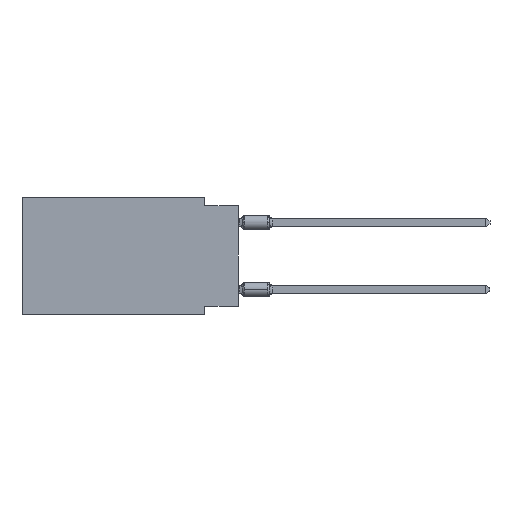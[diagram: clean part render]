
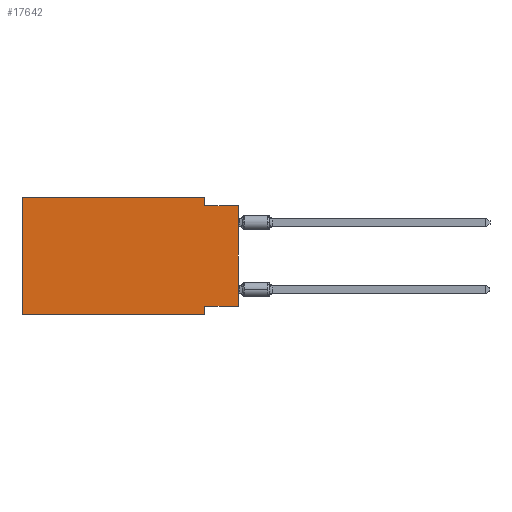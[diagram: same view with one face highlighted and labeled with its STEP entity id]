
A CAD part, left-side view. The second image highlights one B-rep face of the part: STEP entity #17642.
In plain terms, the highlighted planar face has unit normal (-1, 0, 0).
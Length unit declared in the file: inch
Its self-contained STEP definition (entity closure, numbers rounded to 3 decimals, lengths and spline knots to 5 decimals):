
#268 = VECTOR ( 'NONE', #18436, 39.37008 ) ;
#1188 = CARTESIAN_POINT ( 'NONE',  ( 0., 0.645, -0.35 ) ) ;
#1792 = VECTOR ( 'NONE', #5262, 39.37008 ) ;
#1881 = DIRECTION ( 'NONE',  ( 0., 0., -1. ) ) ;
#2581 = CARTESIAN_POINT ( 'NONE',  ( 0., 0.645, 0. ) ) ;
#3119 = DIRECTION ( 'NONE',  ( 0., -1., 0. ) ) ;
#3482 = ORIENTED_EDGE ( 'NONE', *, *, #6467, .T. ) ;
#3500 = CARTESIAN_POINT ( 'NONE',  ( 0., 0., 0. ) ) ;
#3630 = EDGE_CURVE ( 'NONE', #13139, #17908, #11127, .T. ) ;
#3745 = CARTESIAN_POINT ( 'NONE',  ( 0., 0.645, 0. ) ) ;
#5262 = DIRECTION ( 'NONE',  ( 0., 0., 1. ) ) ;
#5352 = ORIENTED_EDGE ( 'NONE', *, *, #11993, .F. ) ;
#6330 = CARTESIAN_POINT ( 'NONE',  ( 0., 0.1, 0. ) ) ;
#6467 = EDGE_CURVE ( 'NONE', #12580, #21857, #8977, .T. ) ;
#6472 = DIRECTION ( 'NONE',  ( 0., 0., 1. ) ) ;
#6615 = VECTOR ( 'NONE', #6472, 39.37008 ) ;
#6706 = VERTEX_POINT ( 'NONE', #23447 ) ;
#6881 = EDGE_CURVE ( 'NONE', #12580, #21814, #10828, .T. ) ;
#7970 = LINE ( 'NONE', #6330, #20561 ) ;
#8062 = EDGE_CURVE ( 'NONE', #13139, #24578, #14453, .T. ) ;
#8977 = LINE ( 'NONE', #16486, #16970 ) ;
#8992 = ORIENTED_EDGE ( 'NONE', *, *, #3630, .T. ) ;
#9120 = ORIENTED_EDGE ( 'NONE', *, *, #24662, .F. ) ;
#9430 = ORIENTED_EDGE ( 'NONE', *, *, #8062, .F. ) ;
#9650 = DIRECTION ( 'NONE',  ( 0., -1., 0. ) ) ;
#9866 = CARTESIAN_POINT ( 'NONE',  ( 0., 0., -0.025 ) ) ;
#10828 = LINE ( 'NONE', #20180, #6615 ) ;
#10831 = CARTESIAN_POINT ( 'NONE',  ( 0., 0., -0.325 ) ) ;
#10899 = EDGE_LOOP ( 'NONE', ( #8992, #5352, #17950, #16220, #21722, #3482, #9120, #9430 ) ) ;
#11127 = LINE ( 'NONE', #3500, #1792 ) ;
#11604 = EDGE_CURVE ( 'NONE', #21814, #18678, #19053, .T. ) ;
#11606 = DIRECTION ( 'NONE',  ( 1., 0., 0. ) ) ;
#11798 = DIRECTION ( 'NONE',  ( 0., 0., -1. ) ) ;
#11922 = CARTESIAN_POINT ( 'NONE',  ( 0., 0.1, 0. ) ) ;
#11942 = CARTESIAN_POINT ( 'NONE',  ( 0., 0.1, -0.35 ) ) ;
#11993 = EDGE_CURVE ( 'NONE', #6706, #17908, #13275, .T. ) ;
#12474 = EDGE_CURVE ( 'NONE', #18678, #6706, #7970, .T. ) ;
#12580 = VERTEX_POINT ( 'NONE', #1188 ) ;
#12879 = DIRECTION ( 'NONE',  ( 0., 0., -1. ) ) ;
#13128 = PLANE ( 'NONE',  #24532 ) ;
#13139 = VERTEX_POINT ( 'NONE', #17342 ) ;
#13275 = LINE ( 'NONE', #13401, #22960 ) ;
#13401 = CARTESIAN_POINT ( 'NONE',  ( 0., 0., -0.025 ) ) ;
#14453 = LINE ( 'NONE', #10831, #268 ) ;
#16220 = ORIENTED_EDGE ( 'NONE', *, *, #11604, .F. ) ;
#16486 = CARTESIAN_POINT ( 'NONE',  ( 0., 0.645, -0.35 ) ) ;
#16970 = VECTOR ( 'NONE', #3119, 39.37008 ) ;
#17063 = DIRECTION ( 'NONE',  ( 0., -1., 0. ) ) ;
#17342 = CARTESIAN_POINT ( 'NONE',  ( 0., 0., -0.325 ) ) ;
#17642 = ADVANCED_FACE ( 'NONE', ( #20738 ), #13128, .F. ) ;
#17908 = VERTEX_POINT ( 'NONE', #9866 ) ;
#17950 = ORIENTED_EDGE ( 'NONE', *, *, #12474, .F. ) ;
#18436 = DIRECTION ( 'NONE',  ( 0., 1., 0. ) ) ;
#18678 = VERTEX_POINT ( 'NONE', #11922 ) ;
#19053 = LINE ( 'NONE', #20796, #23328 ) ;
#20180 = CARTESIAN_POINT ( 'NONE',  ( 0., 0.645, 0. ) ) ;
#20373 = LINE ( 'NONE', #24253, #22623 ) ;
#20561 = VECTOR ( 'NONE', #11798, 39.37008 ) ;
#20738 = FACE_OUTER_BOUND ( 'NONE', #10899, .T. ) ;
#20796 = CARTESIAN_POINT ( 'NONE',  ( 0., 0.645, 0. ) ) ;
#21722 = ORIENTED_EDGE ( 'NONE', *, *, #6881, .F. ) ;
#21814 = VERTEX_POINT ( 'NONE', #2581 ) ;
#21857 = VERTEX_POINT ( 'NONE', #11942 ) ;
#22623 = VECTOR ( 'NONE', #12879, 39.37008 ) ;
#22960 = VECTOR ( 'NONE', #9650, 39.37008 ) ;
#23328 = VECTOR ( 'NONE', #17063, 39.37008 ) ;
#23447 = CARTESIAN_POINT ( 'NONE',  ( 0., 0.1, -0.025 ) ) ;
#23625 = CARTESIAN_POINT ( 'NONE',  ( 0., 0.1, -0.325 ) ) ;
#24253 = CARTESIAN_POINT ( 'NONE',  ( 0., 0.1, -0.35 ) ) ;
#24532 = AXIS2_PLACEMENT_3D ( 'NONE', #3745, #11606, #1881 ) ;
#24578 = VERTEX_POINT ( 'NONE', #23625 ) ;
#24662 = EDGE_CURVE ( 'NONE', #24578, #21857, #20373, .T. ) ;
